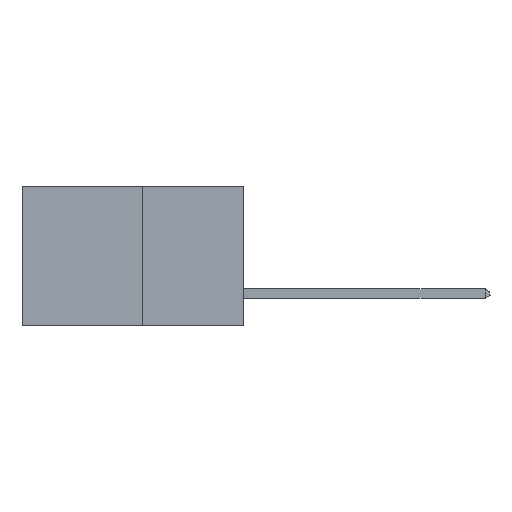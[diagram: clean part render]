
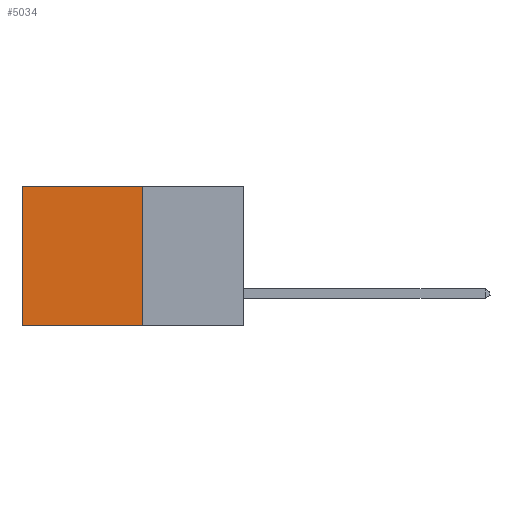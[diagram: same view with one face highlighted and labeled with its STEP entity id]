
A CAD part, left-side view. The second image highlights one B-rep face of the part: STEP entity #5034.
In plain terms, the highlighted planar face has unit normal (-1, 0, 0).
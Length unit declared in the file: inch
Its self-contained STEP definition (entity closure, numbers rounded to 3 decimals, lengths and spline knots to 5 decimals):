
#33 = CARTESIAN_POINT ( 'NONE',  ( 0.277, 0.27, -0.37 ) ) ;
#203 = DIRECTION ( 'NONE',  ( 0., 1., 0. ) ) ;
#372 = VECTOR ( 'NONE', #203, 39.37008 ) ;
#497 = CARTESIAN_POINT ( 'NONE',  ( 0.277, 0.27, 0. ) ) ;
#711 = ORIENTED_EDGE ( 'NONE', *, *, #7700, .F. ) ;
#747 = EDGE_CURVE ( 'NONE', #4581, #4106, #930, .T. ) ;
#772 = VECTOR ( 'NONE', #5367, 39.37008 ) ;
#885 = DIRECTION ( 'NONE',  ( 1., 0., 0. ) ) ;
#911 = ORIENTED_EDGE ( 'NONE', *, *, #2836, .T. ) ;
#930 = LINE ( 'NONE', #497, #4944 ) ;
#1233 = EDGE_LOOP ( 'NONE', ( #911, #711, #3997, #7098 ) ) ;
#2684 = LINE ( 'NONE', #5336, #772 ) ;
#2794 = LINE ( 'NONE', #5789, #372 ) ;
#2836 = EDGE_CURVE ( 'NONE', #4106, #5283, #2684, .T. ) ;
#3869 = CARTESIAN_POINT ( 'NONE',  ( 0.277, 0.27, -0.37 ) ) ;
#3997 = ORIENTED_EDGE ( 'NONE', *, *, #7133, .F. ) ;
#4106 = VERTEX_POINT ( 'NONE', #9986 ) ;
#4247 = DIRECTION ( 'NONE',  ( 0., 0., -1. ) ) ;
#4581 = VERTEX_POINT ( 'NONE', #8292 ) ;
#4885 = PLANE ( 'NONE',  #5461 ) ;
#4944 = VECTOR ( 'NONE', #9288, 39.37008 ) ;
#5034 = ADVANCED_FACE ( 'NONE', ( #8646 ), #4885, .F. ) ;
#5069 = LINE ( 'NONE', #5835, #6912 ) ;
#5283 = VERTEX_POINT ( 'NONE', #9852 ) ;
#5336 = CARTESIAN_POINT ( 'NONE',  ( 0.277, 0.59, -0.37 ) ) ;
#5367 = DIRECTION ( 'NONE',  ( 0., 0., -1. ) ) ;
#5461 = AXIS2_PLACEMENT_3D ( 'NONE', #33, #885, #6441 ) ;
#5789 = CARTESIAN_POINT ( 'NONE',  ( 0.277, 0.27, -0.37 ) ) ;
#5835 = CARTESIAN_POINT ( 'NONE',  ( 0.277, 0.27, -0.37 ) ) ;
#6441 = DIRECTION ( 'NONE',  ( 0., 0., -1. ) ) ;
#6912 = VECTOR ( 'NONE', #4247, 39.37008 ) ;
#7098 = ORIENTED_EDGE ( 'NONE', *, *, #747, .T. ) ;
#7133 = EDGE_CURVE ( 'NONE', #4581, #8751, #5069, .T. ) ;
#7700 = EDGE_CURVE ( 'NONE', #8751, #5283, #2794, .T. ) ;
#8292 = CARTESIAN_POINT ( 'NONE',  ( 0.277, 0.27, 0. ) ) ;
#8646 = FACE_OUTER_BOUND ( 'NONE', #1233, .T. ) ;
#8751 = VERTEX_POINT ( 'NONE', #3869 ) ;
#9288 = DIRECTION ( 'NONE',  ( 0., 1., 0. ) ) ;
#9852 = CARTESIAN_POINT ( 'NONE',  ( 0.277, 0.59, -0.37 ) ) ;
#9986 = CARTESIAN_POINT ( 'NONE',  ( 0.277, 0.59, 0. ) ) ;
